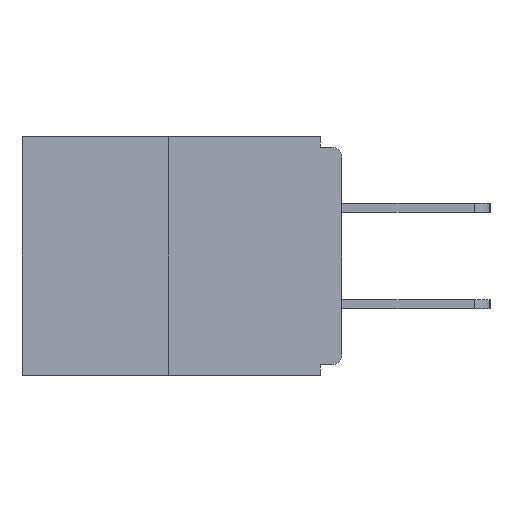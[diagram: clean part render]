
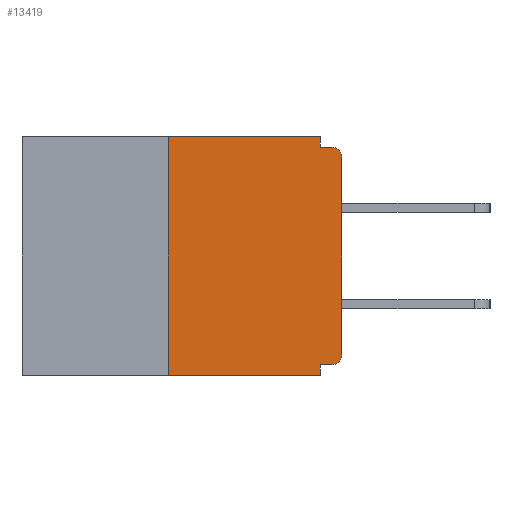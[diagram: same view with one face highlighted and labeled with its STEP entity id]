
A CAD part, left-side view. The second image highlights one B-rep face of the part: STEP entity #13419.
In plain terms, the highlighted planar face has unit normal (-1, 0, 0).
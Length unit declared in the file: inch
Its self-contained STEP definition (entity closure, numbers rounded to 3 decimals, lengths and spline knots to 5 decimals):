
#177 = EDGE_CURVE ( 'NONE', #4415, #27005, #10089, .T. ) ;
#316 = VECTOR ( 'NONE', #19123, 39.37008 ) ;
#390 = DIRECTION ( 'NONE',  ( 0., 0., -1. ) ) ;
#493 = ORIENTED_EDGE ( 'NONE', *, *, #24690, .T. ) ;
#776 = AXIS2_PLACEMENT_3D ( 'NONE', #26702, #13649, #18455 ) ;
#895 = EDGE_CURVE ( 'NONE', #7944, #9129, #4228, .T. ) ;
#989 = CARTESIAN_POINT ( 'NONE',  ( 0., 0.031, -0.343 ) ) ;
#1022 = LINE ( 'NONE', #8981, #11987 ) ;
#1074 = EDGE_CURVE ( 'NONE', #7944, #16099, #2140, .T. ) ;
#1172 = DIRECTION ( 'NONE',  ( 0., -1., 0. ) ) ;
#1678 = CARTESIAN_POINT ( 'NONE',  ( 0., 0.015, -0.03 ) ) ;
#2006 = CIRCLE ( 'NONE', #10897, 0.015 ) ;
#2140 = LINE ( 'NONE', #25405, #27410 ) ;
#3169 = VERTEX_POINT ( 'NONE', #27178 ) ;
#3324 = LINE ( 'NONE', #989, #3660 ) ;
#3434 = VECTOR ( 'NONE', #28131, 39.37008 ) ;
#3660 = VECTOR ( 'NONE', #5209, 39.37008 ) ;
#3797 = DIRECTION ( 'NONE',  ( 0., 0., -1. ) ) ;
#3896 = CARTESIAN_POINT ( 'NONE',  ( 0., 0.015, -0.328 ) ) ;
#4228 = CIRCLE ( 'NONE', #22672, 0.015 ) ;
#4415 = VERTEX_POINT ( 'NONE', #26055 ) ;
#4471 = EDGE_CURVE ( 'NONE', #3169, #16581, #1022, .T. ) ;
#4683 = VERTEX_POINT ( 'NONE', #14012 ) ;
#5209 = DIRECTION ( 'NONE',  ( 0., 0., -1. ) ) ;
#5370 = VECTOR ( 'NONE', #1172, 39.37008 ) ;
#5903 = DIRECTION ( 'NONE',  ( -1., 0., 0. ) ) ;
#6161 = CARTESIAN_POINT ( 'NONE',  ( 0., 0.031, -0.015 ) ) ;
#6360 = EDGE_CURVE ( 'NONE', #16099, #27789, #3324, .T. ) ;
#6596 = CARTESIAN_POINT ( 'NONE',  ( 0., 0.031, -0.328 ) ) ;
#6751 = LINE ( 'NONE', #27351, #5370 ) ;
#7150 = ORIENTED_EDGE ( 'NONE', *, *, #6360, .F. ) ;
#7744 = CARTESIAN_POINT ( 'NONE',  ( 0., 0., -0.03 ) ) ;
#7944 = VERTEX_POINT ( 'NONE', #3896 ) ;
#8396 = DIRECTION ( 'NONE',  ( 0., 0., -1. ) ) ;
#8981 = CARTESIAN_POINT ( 'NONE',  ( 0., 0.25, 0. ) ) ;
#9129 = VERTEX_POINT ( 'NONE', #9706 ) ;
#9706 = CARTESIAN_POINT ( 'NONE',  ( 0., 0., -0.313 ) ) ;
#10089 = LINE ( 'NONE', #21237, #26159 ) ;
#10397 = EDGE_CURVE ( 'NONE', #3169, #27789, #18224, .T. ) ;
#10763 = EDGE_LOOP ( 'NONE', ( #15893, #17619, #20298, #7150, #14307, #22251, #15112, #493, #13244, #27263 ) ) ;
#10897 = AXIS2_PLACEMENT_3D ( 'NONE', #1678, #14889, #8396 ) ;
#11347 = LINE ( 'NONE', #25949, #3434 ) ;
#11987 = VECTOR ( 'NONE', #26139, 39.37008 ) ;
#12223 = VERTEX_POINT ( 'NONE', #7744 ) ;
#13244 = ORIENTED_EDGE ( 'NONE', *, *, #21261, .F. ) ;
#13419 = ADVANCED_FACE ( 'NONE', ( #22822 ), #26431, .F. ) ;
#13649 = DIRECTION ( 'NONE',  ( 1., 0., 0. ) ) ;
#14012 = CARTESIAN_POINT ( 'NONE',  ( 0., 0.015, -0.015 ) ) ;
#14307 = ORIENTED_EDGE ( 'NONE', *, *, #1074, .F. ) ;
#14477 = VECTOR ( 'NONE', #18482, 39.37008 ) ;
#14511 = CARTESIAN_POINT ( 'NONE',  ( 0., 0.031, -0.343 ) ) ;
#14889 = DIRECTION ( 'NONE',  ( -1., 0., 0. ) ) ;
#15112 = ORIENTED_EDGE ( 'NONE', *, *, #24113, .T. ) ;
#15893 = ORIENTED_EDGE ( 'NONE', *, *, #25826, .F. ) ;
#16099 = VERTEX_POINT ( 'NONE', #6596 ) ;
#16581 = VERTEX_POINT ( 'NONE', #20198 ) ;
#16734 = LINE ( 'NONE', #23513, #316 ) ;
#16793 = CARTESIAN_POINT ( 'NONE',  ( 0., 0.015, -0.313 ) ) ;
#17619 = ORIENTED_EDGE ( 'NONE', *, *, #4471, .F. ) ;
#18224 = LINE ( 'NONE', #18567, #14477 ) ;
#18455 = DIRECTION ( 'NONE',  ( 0., 0., -1. ) ) ;
#18482 = DIRECTION ( 'NONE',  ( 0., -1., 0. ) ) ;
#18567 = CARTESIAN_POINT ( 'NONE',  ( 0., 0.46, -0.343 ) ) ;
#19123 = DIRECTION ( 'NONE',  ( 0., 0., 1. ) ) ;
#20198 = CARTESIAN_POINT ( 'NONE',  ( 0., 0.25, 0. ) ) ;
#20298 = ORIENTED_EDGE ( 'NONE', *, *, #10397, .T. ) ;
#21237 = CARTESIAN_POINT ( 'NONE',  ( 0., 0.031, 0. ) ) ;
#21261 = EDGE_CURVE ( 'NONE', #27005, #4683, #11347, .T. ) ;
#22251 = ORIENTED_EDGE ( 'NONE', *, *, #895, .T. ) ;
#22672 = AXIS2_PLACEMENT_3D ( 'NONE', #16793, #5903, #3797 ) ;
#22822 = FACE_OUTER_BOUND ( 'NONE', #10763, .T. ) ;
#23513 = CARTESIAN_POINT ( 'NONE',  ( 0., 0., 0. ) ) ;
#24113 = EDGE_CURVE ( 'NONE', #9129, #12223, #16734, .T. ) ;
#24690 = EDGE_CURVE ( 'NONE', #12223, #4683, #2006, .T. ) ;
#25405 = CARTESIAN_POINT ( 'NONE',  ( 0., 0., -0.328 ) ) ;
#25826 = EDGE_CURVE ( 'NONE', #16581, #4415, #6751, .T. ) ;
#25949 = CARTESIAN_POINT ( 'NONE',  ( 0., 0., -0.015 ) ) ;
#26055 = CARTESIAN_POINT ( 'NONE',  ( 0., 0.031, 0. ) ) ;
#26139 = DIRECTION ( 'NONE',  ( 0., 0., 1. ) ) ;
#26159 = VECTOR ( 'NONE', #390, 39.37008 ) ;
#26431 = PLANE ( 'NONE',  #776 ) ;
#26702 = CARTESIAN_POINT ( 'NONE',  ( 0., 0.46, 0. ) ) ;
#27005 = VERTEX_POINT ( 'NONE', #6161 ) ;
#27178 = CARTESIAN_POINT ( 'NONE',  ( 0., 0.25, -0.343 ) ) ;
#27263 = ORIENTED_EDGE ( 'NONE', *, *, #177, .F. ) ;
#27351 = CARTESIAN_POINT ( 'NONE',  ( 0., 0.46, 0. ) ) ;
#27410 = VECTOR ( 'NONE', #27729, 39.37008 ) ;
#27729 = DIRECTION ( 'NONE',  ( 0., 1., 0. ) ) ;
#27789 = VERTEX_POINT ( 'NONE', #14511 ) ;
#28131 = DIRECTION ( 'NONE',  ( 0., -1., 0. ) ) ;
